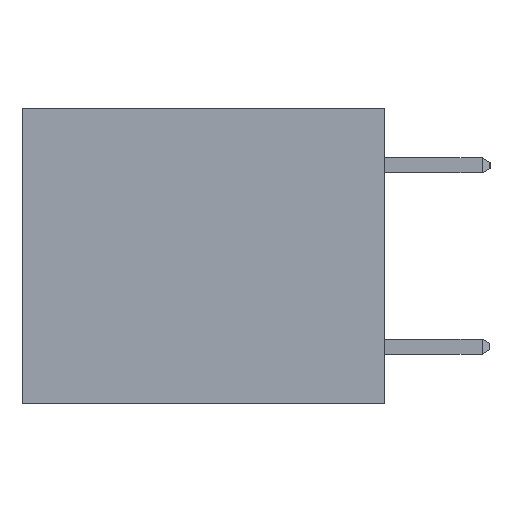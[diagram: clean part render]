
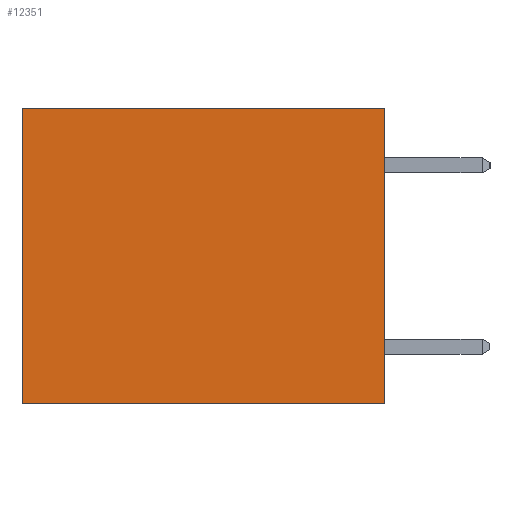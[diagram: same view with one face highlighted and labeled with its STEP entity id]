
A CAD part, left-side view. The second image highlights one B-rep face of the part: STEP entity #12351.
In plain terms, the highlighted planar face has unit normal (-1, 0, 0).
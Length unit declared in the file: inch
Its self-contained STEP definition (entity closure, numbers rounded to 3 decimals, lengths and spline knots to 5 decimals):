
#83 = CARTESIAN_POINT ( 'NONE',  ( 0.3165, 0., 0. ) ) ;
#257 = PLANE ( 'NONE',  #453 ) ;
#453 = AXIS2_PLACEMENT_3D ( 'NONE', #2878, #4018, #6346 ) ;
#829 = VECTOR ( 'NONE', #14625, 39.37008 ) ;
#1447 = EDGE_LOOP ( 'NONE', ( #3878, #11390, #9271, #10599 ) ) ;
#1572 = LINE ( 'NONE', #83, #13534 ) ;
#2035 = VERTEX_POINT ( 'NONE', #14168 ) ;
#2308 = EDGE_CURVE ( 'NONE', #13462, #14222, #7457, .T. ) ;
#2878 = CARTESIAN_POINT ( 'NONE',  ( 0.3165, 0., -0.49 ) ) ;
#3658 = LINE ( 'NONE', #13058, #9818 ) ;
#3878 = ORIENTED_EDGE ( 'NONE', *, *, #4989, .T. ) ;
#4018 = DIRECTION ( 'NONE',  ( 1., 0., 0. ) ) ;
#4989 = EDGE_CURVE ( 'NONE', #14884, #2035, #6063, .T. ) ;
#5040 = VECTOR ( 'NONE', #14170, 39.37008 ) ;
#6063 = LINE ( 'NONE', #6256, #829 ) ;
#6256 = CARTESIAN_POINT ( 'NONE',  ( 0.3165, 0.6, -0.49 ) ) ;
#6346 = DIRECTION ( 'NONE',  ( 0., 0., -1. ) ) ;
#7355 = CARTESIAN_POINT ( 'NONE',  ( 0.3165, 0.6, 0. ) ) ;
#7457 = LINE ( 'NONE', #9372, #5040 ) ;
#8168 = CARTESIAN_POINT ( 'NONE',  ( 0.3165, 0., 0. ) ) ;
#9102 = EDGE_CURVE ( 'NONE', #14222, #2035, #3658, .T. ) ;
#9271 = ORIENTED_EDGE ( 'NONE', *, *, #2308, .F. ) ;
#9372 = CARTESIAN_POINT ( 'NONE',  ( 0.3165, 0., -0.49 ) ) ;
#9686 = DIRECTION ( 'NONE',  ( 0., 1., 0. ) ) ;
#9818 = VECTOR ( 'NONE', #12007, 39.37008 ) ;
#10335 = EDGE_CURVE ( 'NONE', #13462, #14884, #1572, .T. ) ;
#10413 = CARTESIAN_POINT ( 'NONE',  ( 0.3165, 0., -0.49 ) ) ;
#10599 = ORIENTED_EDGE ( 'NONE', *, *, #10335, .T. ) ;
#11390 = ORIENTED_EDGE ( 'NONE', *, *, #9102, .F. ) ;
#12007 = DIRECTION ( 'NONE',  ( 0., 1., 0. ) ) ;
#12351 = ADVANCED_FACE ( 'NONE', ( #13216 ), #257, .F. ) ;
#13058 = CARTESIAN_POINT ( 'NONE',  ( 0.3165, 0., -0.49 ) ) ;
#13216 = FACE_OUTER_BOUND ( 'NONE', #1447, .T. ) ;
#13462 = VERTEX_POINT ( 'NONE', #8168 ) ;
#13534 = VECTOR ( 'NONE', #9686, 39.37008 ) ;
#14168 = CARTESIAN_POINT ( 'NONE',  ( 0.3165, 0.6, -0.49 ) ) ;
#14170 = DIRECTION ( 'NONE',  ( 0., 0., -1. ) ) ;
#14222 = VERTEX_POINT ( 'NONE', #10413 ) ;
#14625 = DIRECTION ( 'NONE',  ( 0., 0., -1. ) ) ;
#14884 = VERTEX_POINT ( 'NONE', #7355 ) ;
